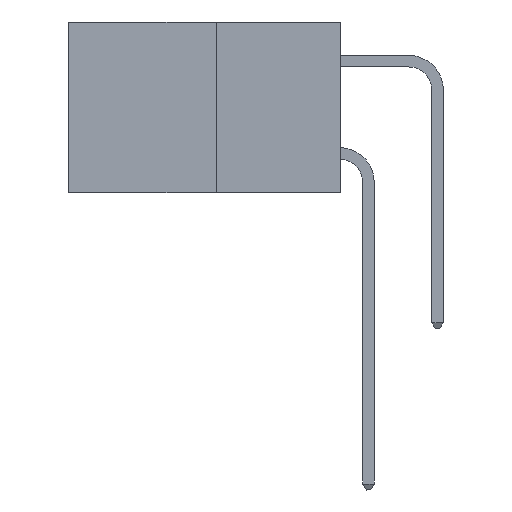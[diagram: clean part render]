
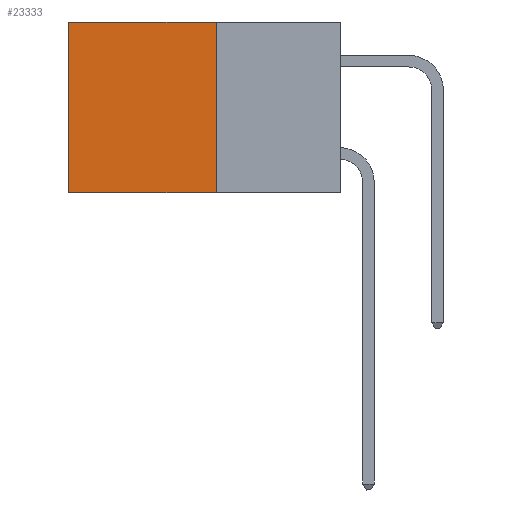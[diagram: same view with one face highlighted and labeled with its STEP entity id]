
A CAD part, left-side view. The second image highlights one B-rep face of the part: STEP entity #23333.
In plain terms, the highlighted planar face has unit normal (-1, 0, 0).
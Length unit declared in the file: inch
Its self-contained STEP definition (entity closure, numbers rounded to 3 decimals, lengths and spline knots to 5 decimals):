
#2 = EDGE_CURVE ( 'NONE', #22732, #18996, #4685, .T. ) ;
#977 = DIRECTION ( 'NONE',  ( 1., 0., 0. ) ) ;
#1184 = DIRECTION ( 'NONE',  ( 0., 0., -1. ) ) ;
#2569 = CARTESIAN_POINT ( 'NONE',  ( 0.277, 0.27, 0. ) ) ;
#2836 = CARTESIAN_POINT ( 'NONE',  ( 0.277, 0.27, -0.37 ) ) ;
#4082 = VECTOR ( 'NONE', #15996, 39.37008 ) ;
#4685 = LINE ( 'NONE', #19621, #4082 ) ;
#5059 = DIRECTION ( 'NONE',  ( 0., 1., 0. ) ) ;
#5275 = AXIS2_PLACEMENT_3D ( 'NONE', #12797, #977, #14746 ) ;
#5598 = LINE ( 'NONE', #10971, #20515 ) ;
#6236 = EDGE_CURVE ( 'NONE', #13896, #18996, #22581, .T. ) ;
#8094 = ORIENTED_EDGE ( 'NONE', *, *, #6236, .F. ) ;
#8901 = PLANE ( 'NONE',  #5275 ) ;
#10083 = EDGE_LOOP ( 'NONE', ( #19877, #8094, #12736, #11536 ) ) ;
#10971 = CARTESIAN_POINT ( 'NONE',  ( 0.277, 0.27, -0.37 ) ) ;
#11536 = ORIENTED_EDGE ( 'NONE', *, *, #20060, .T. ) ;
#12736 = ORIENTED_EDGE ( 'NONE', *, *, #19780, .F. ) ;
#12797 = CARTESIAN_POINT ( 'NONE',  ( 0.277, 0.27, -0.37 ) ) ;
#13896 = VERTEX_POINT ( 'NONE', #2836 ) ;
#14746 = DIRECTION ( 'NONE',  ( 0., 0., -1. ) ) ;
#14847 = CARTESIAN_POINT ( 'NONE',  ( 0.277, 0.27, 0. ) ) ;
#15996 = DIRECTION ( 'NONE',  ( 0., 0., -1. ) ) ;
#16138 = FACE_OUTER_BOUND ( 'NONE', #10083, .T. ) ;
#16739 = CARTESIAN_POINT ( 'NONE',  ( 0.277, 0.27, -0.37 ) ) ;
#18435 = VERTEX_POINT ( 'NONE', #14847 ) ;
#18996 = VERTEX_POINT ( 'NONE', #22270 ) ;
#19572 = VECTOR ( 'NONE', #5059, 39.37008 ) ;
#19621 = CARTESIAN_POINT ( 'NONE',  ( 0.277, 0.59, -0.37 ) ) ;
#19780 = EDGE_CURVE ( 'NONE', #18435, #13896, #5598, .T. ) ;
#19877 = ORIENTED_EDGE ( 'NONE', *, *, #2, .T. ) ;
#20060 = EDGE_CURVE ( 'NONE', #18435, #22732, #20800, .T. ) ;
#20515 = VECTOR ( 'NONE', #1184, 39.37008 ) ;
#20800 = LINE ( 'NONE', #2569, #24682 ) ;
#22100 = DIRECTION ( 'NONE',  ( 0., 1., 0. ) ) ;
#22155 = CARTESIAN_POINT ( 'NONE',  ( 0.277, 0.59, 0. ) ) ;
#22270 = CARTESIAN_POINT ( 'NONE',  ( 0.277, 0.59, -0.37 ) ) ;
#22581 = LINE ( 'NONE', #16739, #19572 ) ;
#22732 = VERTEX_POINT ( 'NONE', #22155 ) ;
#23333 = ADVANCED_FACE ( 'NONE', ( #16138 ), #8901, .F. ) ;
#24682 = VECTOR ( 'NONE', #22100, 39.37008 ) ;
